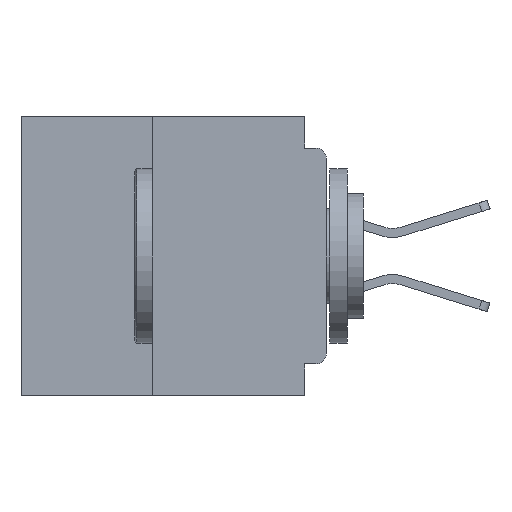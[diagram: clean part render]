
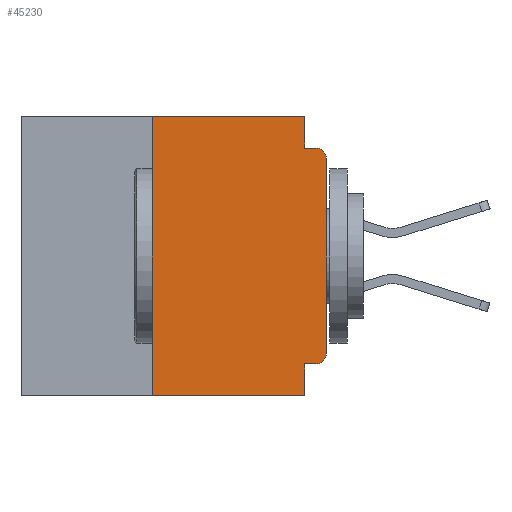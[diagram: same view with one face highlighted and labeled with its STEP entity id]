
A CAD part, left-side view. The second image highlights one B-rep face of the part: STEP entity #45230.
In plain terms, the highlighted planar face has unit normal (-1, 0, 0).
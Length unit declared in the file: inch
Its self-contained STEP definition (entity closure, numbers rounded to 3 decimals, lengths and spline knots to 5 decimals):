
#261 = VERTEX_POINT ( 'NONE', #27048 ) ;
#283 = LINE ( 'NONE', #31044, #20510 ) ;
#798 = CARTESIAN_POINT ( 'NONE',  ( 0., 0.031, 0. ) ) ;
#1665 = ORIENTED_EDGE ( 'NONE', *, *, #2979, .F. ) ;
#2979 = EDGE_CURVE ( 'NONE', #11701, #19457, #21477, .T. ) ;
#6470 = VERTEX_POINT ( 'NONE', #9778 ) ;
#6662 = DIRECTION ( 'NONE',  ( 0., 1., 0. ) ) ;
#8252 = ORIENTED_EDGE ( 'NONE', *, *, #48196, .F. ) ;
#8969 = CARTESIAN_POINT ( 'NONE',  ( 0., 0.25, -0.4 ) ) ;
#9179 = DIRECTION ( 'NONE',  ( -1., 0., 0. ) ) ;
#9778 = CARTESIAN_POINT ( 'NONE',  ( 0., 0.015, -0.355 ) ) ;
#10222 = VECTOR ( 'NONE', #20373, 39.37008 ) ;
#10678 = ORIENTED_EDGE ( 'NONE', *, *, #15951, .F. ) ;
#11470 = VECTOR ( 'NONE', #6662, 39.37008 ) ;
#11701 = VERTEX_POINT ( 'NONE', #32166 ) ;
#12040 = VECTOR ( 'NONE', #16804, 39.37008 ) ;
#12484 = EDGE_CURVE ( 'NONE', #6470, #41160, #51607, .T. ) ;
#12635 = ORIENTED_EDGE ( 'NONE', *, *, #26817, .F. ) ;
#12736 = LINE ( 'NONE', #18678, #11470 ) ;
#13674 = VERTEX_POINT ( 'NONE', #37082 ) ;
#15951 = EDGE_CURVE ( 'NONE', #19457, #37946, #24044, .T. ) ;
#16280 = CARTESIAN_POINT ( 'NONE',  ( 0., 0., -0.045 ) ) ;
#16804 = DIRECTION ( 'NONE',  ( 0., 0., -1. ) ) ;
#17260 = CARTESIAN_POINT ( 'NONE',  ( 0., 0.25, -0.4 ) ) ;
#18184 = AXIS2_PLACEMENT_3D ( 'NONE', #36157, #48172, #24221 ) ;
#18548 = VERTEX_POINT ( 'NONE', #27028 ) ;
#18678 = CARTESIAN_POINT ( 'NONE',  ( 0., 0., -0.355 ) ) ;
#18814 = VERTEX_POINT ( 'NONE', #8969 ) ;
#19021 = CIRCLE ( 'NONE', #26210, 0.015 ) ;
#19428 = VECTOR ( 'NONE', #40021, 39.37008 ) ;
#19457 = VERTEX_POINT ( 'NONE', #798 ) ;
#19672 = VECTOR ( 'NONE', #34904, 39.37008 ) ;
#20373 = DIRECTION ( 'NONE',  ( 0., -1., 0. ) ) ;
#20510 = VECTOR ( 'NONE', #50918, 39.37008 ) ;
#20665 = LINE ( 'NONE', #27971, #19428 ) ;
#20920 = ORIENTED_EDGE ( 'NONE', *, *, #33398, .F. ) ;
#21034 = DIRECTION ( 'NONE',  ( -1., 0., 0. ) ) ;
#21207 = ORIENTED_EDGE ( 'NONE', *, *, #23629, .T. ) ;
#21477 = LINE ( 'NONE', #47740, #42771 ) ;
#23629 = EDGE_CURVE ( 'NONE', #41160, #18548, #20665, .T. ) ;
#24044 = LINE ( 'NONE', #40864, #12040 ) ;
#24221 = DIRECTION ( 'NONE',  ( 0., 0., -1. ) ) ;
#24468 = ORIENTED_EDGE ( 'NONE', *, *, #43096, .T. ) ;
#26210 = AXIS2_PLACEMENT_3D ( 'NONE', #33299, #9179, #37337 ) ;
#26817 = EDGE_CURVE ( 'NONE', #18814, #11701, #40399, .T. ) ;
#27028 = CARTESIAN_POINT ( 'NONE',  ( 0., 0., -0.06 ) ) ;
#27048 = CARTESIAN_POINT ( 'NONE',  ( 0., 0.015, -0.045 ) ) ;
#27053 = EDGE_CURVE ( 'NONE', #6470, #33587, #12736, .T. ) ;
#27971 = CARTESIAN_POINT ( 'NONE',  ( 0., 0., 0. ) ) ;
#30353 = ORIENTED_EDGE ( 'NONE', *, *, #12484, .T. ) ;
#30898 = ORIENTED_EDGE ( 'NONE', *, *, #27053, .F. ) ;
#30906 = CARTESIAN_POINT ( 'NONE',  ( 0., 0.437, -0.4 ) ) ;
#31044 = CARTESIAN_POINT ( 'NONE',  ( 0., 0.031, -0.4 ) ) ;
#31055 = VECTOR ( 'NONE', #45294, 39.37008 ) ;
#32166 = CARTESIAN_POINT ( 'NONE',  ( 0., 0.25, 0. ) ) ;
#33299 = CARTESIAN_POINT ( 'NONE',  ( 0., 0.015, -0.06 ) ) ;
#33398 = EDGE_CURVE ( 'NONE', #37946, #261, #42273, .T. ) ;
#33587 = VERTEX_POINT ( 'NONE', #45402 ) ;
#34904 = DIRECTION ( 'NONE',  ( 0., -1., 0. ) ) ;
#34970 = AXIS2_PLACEMENT_3D ( 'NONE', #45014, #21034, #49022 ) ;
#36157 = CARTESIAN_POINT ( 'NONE',  ( 0., 0.437, 0. ) ) ;
#36876 = ORIENTED_EDGE ( 'NONE', *, *, #42858, .T. ) ;
#37082 = CARTESIAN_POINT ( 'NONE',  ( 0., 0.031, -0.4 ) ) ;
#37337 = DIRECTION ( 'NONE',  ( 0., 0., -1. ) ) ;
#37946 = VERTEX_POINT ( 'NONE', #38348 ) ;
#38348 = CARTESIAN_POINT ( 'NONE',  ( 0., 0.031, -0.045 ) ) ;
#40021 = DIRECTION ( 'NONE',  ( 0., 0., 1. ) ) ;
#40399 = LINE ( 'NONE', #17260, #31055 ) ;
#40864 = CARTESIAN_POINT ( 'NONE',  ( 0., 0.031, 0. ) ) ;
#41160 = VERTEX_POINT ( 'NONE', #51815 ) ;
#41960 = EDGE_LOOP ( 'NONE', ( #21207, #24468, #20920, #10678, #1665, #12635, #36876, #8252, #30898, #30353 ) ) ;
#42273 = LINE ( 'NONE', #16280, #10222 ) ;
#42771 = VECTOR ( 'NONE', #49888, 39.37008 ) ;
#42858 = EDGE_CURVE ( 'NONE', #18814, #13674, #51600, .T. ) ;
#43096 = EDGE_CURVE ( 'NONE', #18548, #261, #19021, .T. ) ;
#45014 = CARTESIAN_POINT ( 'NONE',  ( 0., 0.015, -0.34 ) ) ;
#45230 = ADVANCED_FACE ( 'NONE', ( #45783 ), #52017, .F. ) ;
#45294 = DIRECTION ( 'NONE',  ( 0., 0., 1. ) ) ;
#45402 = CARTESIAN_POINT ( 'NONE',  ( 0., 0.031, -0.355 ) ) ;
#45783 = FACE_OUTER_BOUND ( 'NONE', #41960, .T. ) ;
#47740 = CARTESIAN_POINT ( 'NONE',  ( 0., 0.437, 0. ) ) ;
#48172 = DIRECTION ( 'NONE',  ( 1., 0., 0. ) ) ;
#48196 = EDGE_CURVE ( 'NONE', #33587, #13674, #283, .T. ) ;
#49022 = DIRECTION ( 'NONE',  ( 0., 0., -1. ) ) ;
#49888 = DIRECTION ( 'NONE',  ( 0., -1., 0. ) ) ;
#50918 = DIRECTION ( 'NONE',  ( 0., 0., -1. ) ) ;
#51600 = LINE ( 'NONE', #30906, #19672 ) ;
#51607 = CIRCLE ( 'NONE', #34970, 0.015 ) ;
#51815 = CARTESIAN_POINT ( 'NONE',  ( 0., 0., -0.34 ) ) ;
#52017 = PLANE ( 'NONE',  #18184 ) ;
